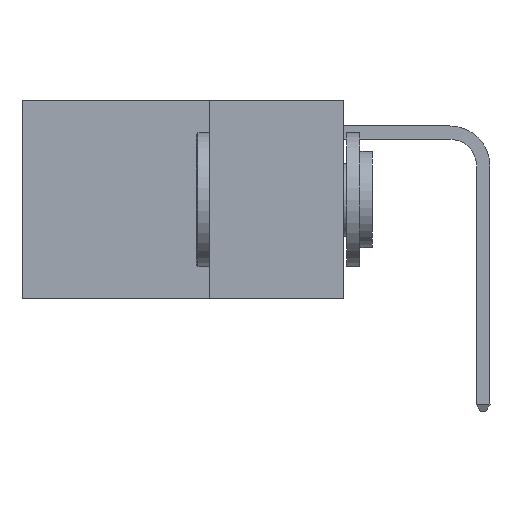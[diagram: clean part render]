
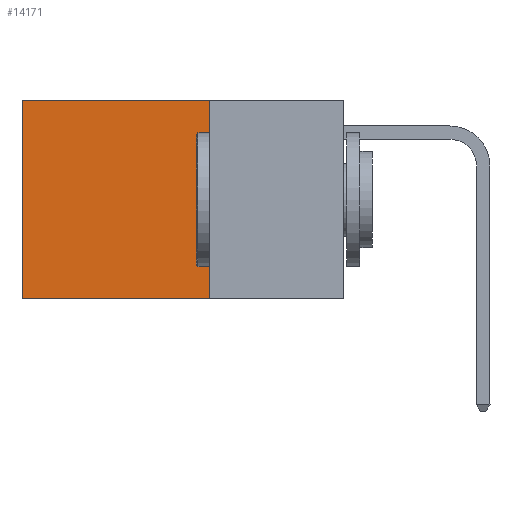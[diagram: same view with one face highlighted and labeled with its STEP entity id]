
A CAD part, left-side view. The second image highlights one B-rep face of the part: STEP entity #14171.
In plain terms, the highlighted planar face has unit normal (-1, 0, 0).
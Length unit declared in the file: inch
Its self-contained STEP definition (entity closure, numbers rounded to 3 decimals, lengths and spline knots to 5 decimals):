
#50 = CARTESIAN_POINT ( 'NONE',  ( 0.2625, 0.25, -0.37 ) ) ;
#578 = VECTOR ( 'NONE', #10145, 39.37008 ) ;
#627 = EDGE_CURVE ( 'NONE', #14947, #8865, #8339, .T. ) ;
#800 = DIRECTION ( 'NONE',  ( 0., 0., -1. ) ) ;
#809 = CARTESIAN_POINT ( 'NONE',  ( 0.2625, 0.25, -0.37 ) ) ;
#1310 = EDGE_CURVE ( 'NONE', #3324, #14947, #1843, .T. ) ;
#1843 = LINE ( 'NONE', #14456, #8012 ) ;
#2553 = PLANE ( 'NONE',  #13225 ) ;
#3324 = VERTEX_POINT ( 'NONE', #6652 ) ;
#3727 = CARTESIAN_POINT ( 'NONE',  ( 0.2625, 0.25, 0. ) ) ;
#4665 = CARTESIAN_POINT ( 'NONE',  ( 0.2625, 0.6, 0. ) ) ;
#5035 = CARTESIAN_POINT ( 'NONE',  ( 0.2625, 0.25, 0. ) ) ;
#5955 = CARTESIAN_POINT ( 'NONE',  ( 0.2625, 0.6, 0. ) ) ;
#6652 = CARTESIAN_POINT ( 'NONE',  ( 0.2625, 0.25, 0. ) ) ;
#7345 = DIRECTION ( 'NONE',  ( 0., 1., 0. ) ) ;
#7368 = EDGE_LOOP ( 'NONE', ( #16493, #8860, #8343, #11022 ) ) ;
#8012 = VECTOR ( 'NONE', #9698, 39.37008 ) ;
#8128 = FACE_OUTER_BOUND ( 'NONE', #7368, .T. ) ;
#8339 = LINE ( 'NONE', #809, #11107 ) ;
#8343 = ORIENTED_EDGE ( 'NONE', *, *, #1310, .F. ) ;
#8836 = EDGE_CURVE ( 'NONE', #3324, #13396, #11385, .T. ) ;
#8860 = ORIENTED_EDGE ( 'NONE', *, *, #627, .F. ) ;
#8865 = VERTEX_POINT ( 'NONE', #14044 ) ;
#9698 = DIRECTION ( 'NONE',  ( 0., 0., -1. ) ) ;
#10014 = EDGE_CURVE ( 'NONE', #13396, #8865, #11093, .T. ) ;
#10145 = DIRECTION ( 'NONE',  ( 0., 1., 0. ) ) ;
#11022 = ORIENTED_EDGE ( 'NONE', *, *, #8836, .T. ) ;
#11093 = LINE ( 'NONE', #4665, #15565 ) ;
#11107 = VECTOR ( 'NONE', #7345, 39.37008 ) ;
#11385 = LINE ( 'NONE', #5035, #578 ) ;
#11413 = DIRECTION ( 'NONE',  ( 1., 0., 0. ) ) ;
#11724 = DIRECTION ( 'NONE',  ( 0., 0., -1. ) ) ;
#13225 = AXIS2_PLACEMENT_3D ( 'NONE', #3727, #11413, #11724 ) ;
#13396 = VERTEX_POINT ( 'NONE', #5955 ) ;
#14044 = CARTESIAN_POINT ( 'NONE',  ( 0.2625, 0.6, -0.37 ) ) ;
#14171 = ADVANCED_FACE ( 'NONE', ( #8128 ), #2553, .F. ) ;
#14456 = CARTESIAN_POINT ( 'NONE',  ( 0.2625, 0.25, 0. ) ) ;
#14947 = VERTEX_POINT ( 'NONE', #50 ) ;
#15565 = VECTOR ( 'NONE', #800, 39.37008 ) ;
#16493 = ORIENTED_EDGE ( 'NONE', *, *, #10014, .T. ) ;
